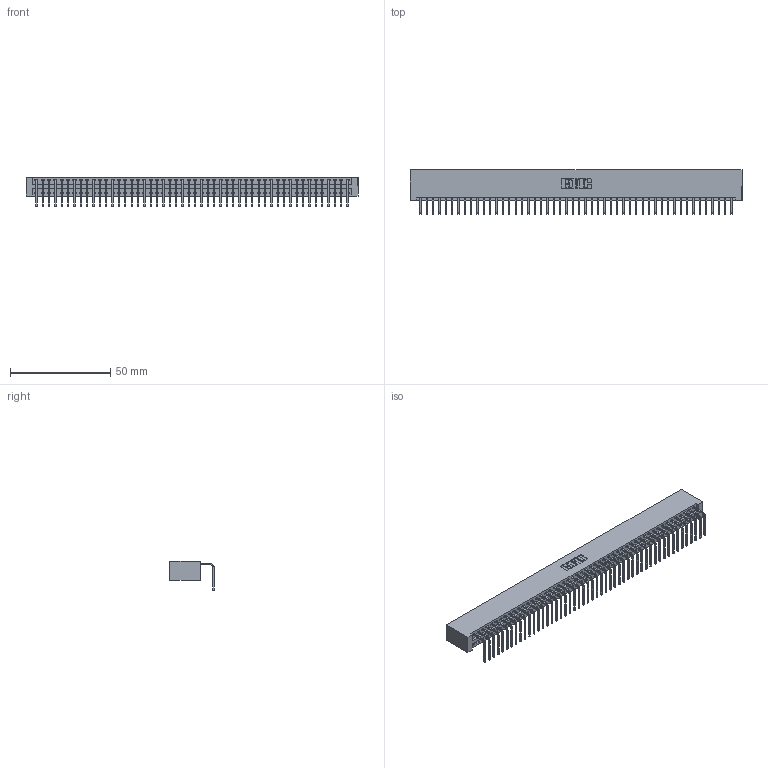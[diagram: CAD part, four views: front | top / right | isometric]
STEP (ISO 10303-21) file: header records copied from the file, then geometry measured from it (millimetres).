
FILE_DESCRIPTION (( 'STEP AP203' ), '1' );
FILE_NAME ('346-050-558-101.STEP', '2022-05-10T03:59:40', ( '' ), ( '' ), 'SwSTEP 2.0', 'SolidWorks 2020', '' );
FILE_SCHEMA (( 'CONFIG_CONTROL_DESIGN' ));
Length unit declared in the file: inch
Products named in the file (3): 345-292-001_558 Tail - 2; 346 Part_No Mounting Lugs; 346-050-558-101
Assembly tree (51 placements, depth 2):
  346-050-558-101
    346 Part_No Mounting Lugs
    345-292-001_558 Tail - 2  x50
Bounding box: 165.99 x 22.16 x 14.73 mm (x, y, z)
Volume: 16659.9 mm3; surface area: 21978 mm2
Topology: 51 solids, 51 shells, 3114 faces, 9405 edges, 6202 vertices
Faces by surface type: plane 2172, cylinder 942
Entity records: 29761 total; most frequent: CARTESIAN_POINT 5106, ORIENTED_EDGE 5090, DIRECTION 4489, EDGE_CURVE 2545, LINE 2221, VECTOR 2221, VERTEX_POINT 1694, AXIS2_PLACEMENT_3D 1134
